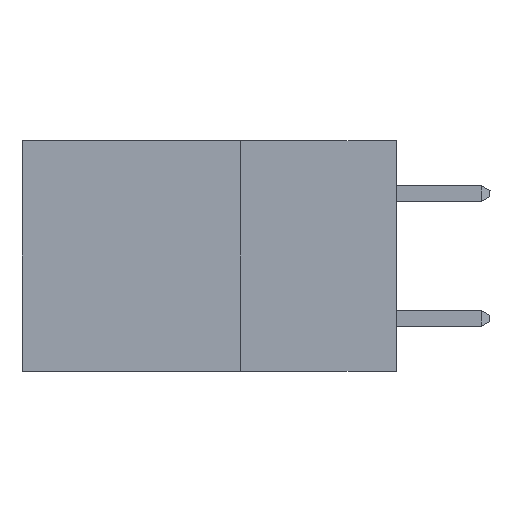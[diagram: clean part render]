
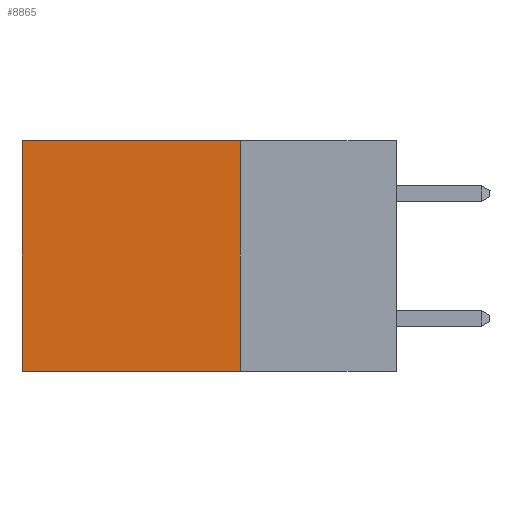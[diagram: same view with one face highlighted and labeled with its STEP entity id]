
A CAD part, left-side view. The second image highlights one B-rep face of the part: STEP entity #8865.
In plain terms, the highlighted planar face has unit normal (-1, 0, 0).
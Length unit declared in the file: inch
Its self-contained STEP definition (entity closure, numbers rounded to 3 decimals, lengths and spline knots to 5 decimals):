
#352 = AXIS2_PLACEMENT_3D ( 'NONE', #6417, #1680, #7165 ) ;
#851 = PLANE ( 'NONE',  #352 ) ;
#1262 = CARTESIAN_POINT ( 'NONE',  ( 0.298, 0.25, -0.37 ) ) ;
#1680 = DIRECTION ( 'NONE',  ( 1., 0., 0. ) ) ;
#2147 = CARTESIAN_POINT ( 'NONE',  ( 0.298, 0.6, -0.37 ) ) ;
#2806 = CARTESIAN_POINT ( 'NONE',  ( 0.298, 0.25, 0. ) ) ;
#2905 = DIRECTION ( 'NONE',  ( 0., 0., -1. ) ) ;
#2937 = CARTESIAN_POINT ( 'NONE',  ( 0.298, 0.25, -0.37 ) ) ;
#3413 = CARTESIAN_POINT ( 'NONE',  ( 0.298, 0.25, 0. ) ) ;
#3952 = VECTOR ( 'NONE', #6002, 39.37008 ) ;
#4022 = ORIENTED_EDGE ( 'NONE', *, *, #8852, .T. ) ;
#4044 = DIRECTION ( 'NONE',  ( 0., 0., -1. ) ) ;
#4609 = EDGE_LOOP ( 'NONE', ( #4022, #6537, #7810, #7365 ) ) ;
#4799 = LINE ( 'NONE', #8401, #5298 ) ;
#4956 = FACE_OUTER_BOUND ( 'NONE', #4609, .T. ) ;
#5128 = DIRECTION ( 'NONE',  ( 0., 1., 0. ) ) ;
#5215 = VECTOR ( 'NONE', #4044, 39.37008 ) ;
#5298 = VECTOR ( 'NONE', #5128, 39.37008 ) ;
#6002 = DIRECTION ( 'NONE',  ( 0., 1., 0. ) ) ;
#6038 = EDGE_CURVE ( 'NONE', #9598, #6357, #4799, .T. ) ;
#6288 = LINE ( 'NONE', #1262, #3952 ) ;
#6357 = VERTEX_POINT ( 'NONE', #8797 ) ;
#6417 = CARTESIAN_POINT ( 'NONE',  ( 0.298, 0.25, 0. ) ) ;
#6537 = ORIENTED_EDGE ( 'NONE', *, *, #9826, .F. ) ;
#7022 = LINE ( 'NONE', #8609, #5215 ) ;
#7037 = LINE ( 'NONE', #2806, #7253 ) ;
#7165 = DIRECTION ( 'NONE',  ( 0., 0., -1. ) ) ;
#7253 = VECTOR ( 'NONE', #2905, 39.37008 ) ;
#7352 = EDGE_CURVE ( 'NONE', #9598, #7677, #7037, .T. ) ;
#7365 = ORIENTED_EDGE ( 'NONE', *, *, #6038, .T. ) ;
#7677 = VERTEX_POINT ( 'NONE', #2937 ) ;
#7810 = ORIENTED_EDGE ( 'NONE', *, *, #7352, .F. ) ;
#8401 = CARTESIAN_POINT ( 'NONE',  ( 0.298, 0.25, 0. ) ) ;
#8609 = CARTESIAN_POINT ( 'NONE',  ( 0.298, 0.6, 0. ) ) ;
#8797 = CARTESIAN_POINT ( 'NONE',  ( 0.298, 0.6, 0. ) ) ;
#8852 = EDGE_CURVE ( 'NONE', #6357, #9841, #7022, .T. ) ;
#8865 = ADVANCED_FACE ( 'NONE', ( #4956 ), #851, .F. ) ;
#9598 = VERTEX_POINT ( 'NONE', #3413 ) ;
#9826 = EDGE_CURVE ( 'NONE', #7677, #9841, #6288, .T. ) ;
#9841 = VERTEX_POINT ( 'NONE', #2147 ) ;
